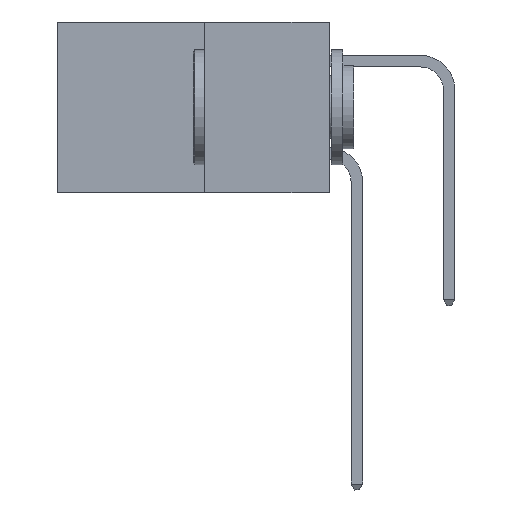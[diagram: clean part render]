
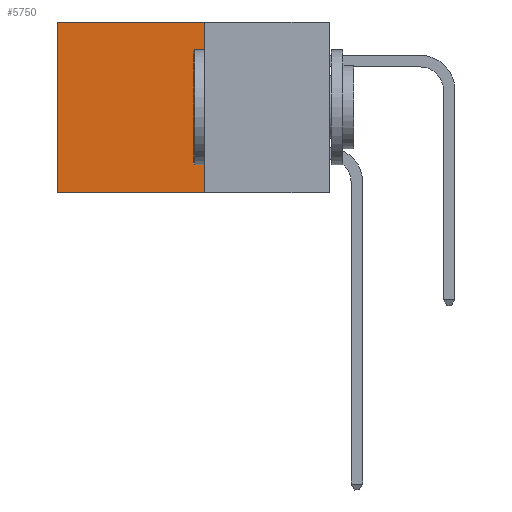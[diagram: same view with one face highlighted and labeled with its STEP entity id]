
A CAD part, left-side view. The second image highlights one B-rep face of the part: STEP entity #5750.
In plain terms, the highlighted planar face has unit normal (-1, 0, 0).
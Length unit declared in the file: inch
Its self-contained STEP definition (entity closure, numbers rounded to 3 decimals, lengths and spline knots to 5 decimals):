
#206 = DIRECTION ( 'NONE',  ( 0., 1., 0. ) ) ;
#980 = VECTOR ( 'NONE', #8989, 39.37008 ) ;
#1050 = CARTESIAN_POINT ( 'NONE',  ( 0.277, 0.59, -0.37 ) ) ;
#1103 = EDGE_LOOP ( 'NONE', ( #7352, #8091, #2078, #6495 ) ) ;
#1198 = DIRECTION ( 'NONE',  ( 1., 0., 0. ) ) ;
#1684 = VECTOR ( 'NONE', #5759, 39.37008 ) ;
#1826 = CARTESIAN_POINT ( 'NONE',  ( 0.277, 0.27, -0.37 ) ) ;
#2078 = ORIENTED_EDGE ( 'NONE', *, *, #2322, .F. ) ;
#2322 = EDGE_CURVE ( 'NONE', #4207, #3701, #5319, .T. ) ;
#2657 = EDGE_CURVE ( 'NONE', #4207, #8148, #6764, .T. ) ;
#3196 = VECTOR ( 'NONE', #206, 39.37008 ) ;
#3701 = VERTEX_POINT ( 'NONE', #1826 ) ;
#4207 = VERTEX_POINT ( 'NONE', #5449 ) ;
#5029 = EDGE_CURVE ( 'NONE', #3701, #9526, #7318, .T. ) ;
#5124 = PLANE ( 'NONE',  #8753 ) ;
#5319 = LINE ( 'NONE', #6371, #9199 ) ;
#5443 = CARTESIAN_POINT ( 'NONE',  ( 0.277, 0.59, -0.37 ) ) ;
#5449 = CARTESIAN_POINT ( 'NONE',  ( 0.277, 0.27, 0. ) ) ;
#5640 = EDGE_CURVE ( 'NONE', #8148, #9526, #10198, .T. ) ;
#5750 = ADVANCED_FACE ( 'NONE', ( #6697 ), #5124, .F. ) ;
#5759 = DIRECTION ( 'NONE',  ( 0., 0., -1. ) ) ;
#5898 = CARTESIAN_POINT ( 'NONE',  ( 0.277, 0.27, -0.37 ) ) ;
#6371 = CARTESIAN_POINT ( 'NONE',  ( 0.277, 0.27, -0.37 ) ) ;
#6423 = CARTESIAN_POINT ( 'NONE',  ( 0.277, 0.59, 0. ) ) ;
#6495 = ORIENTED_EDGE ( 'NONE', *, *, #2657, .T. ) ;
#6682 = DIRECTION ( 'NONE',  ( 0., 0., -1. ) ) ;
#6697 = FACE_OUTER_BOUND ( 'NONE', #1103, .T. ) ;
#6764 = LINE ( 'NONE', #7974, #980 ) ;
#7318 = LINE ( 'NONE', #8128, #3196 ) ;
#7352 = ORIENTED_EDGE ( 'NONE', *, *, #5640, .T. ) ;
#7974 = CARTESIAN_POINT ( 'NONE',  ( 0.277, 0.27, 0. ) ) ;
#8091 = ORIENTED_EDGE ( 'NONE', *, *, #5029, .F. ) ;
#8128 = CARTESIAN_POINT ( 'NONE',  ( 0.277, 0.27, -0.37 ) ) ;
#8148 = VERTEX_POINT ( 'NONE', #6423 ) ;
#8753 = AXIS2_PLACEMENT_3D ( 'NONE', #5898, #1198, #6682 ) ;
#8989 = DIRECTION ( 'NONE',  ( 0., 1., 0. ) ) ;
#9199 = VECTOR ( 'NONE', #9495, 39.37008 ) ;
#9495 = DIRECTION ( 'NONE',  ( 0., 0., -1. ) ) ;
#9526 = VERTEX_POINT ( 'NONE', #5443 ) ;
#10198 = LINE ( 'NONE', #1050, #1684 ) ;
